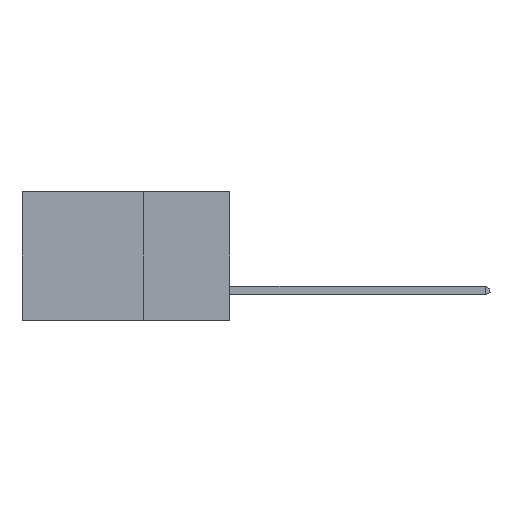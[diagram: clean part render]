
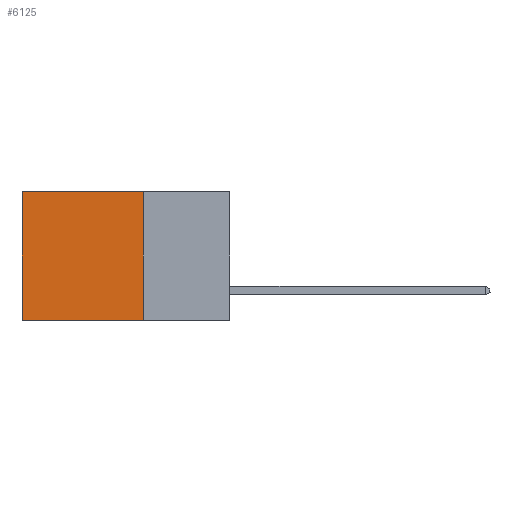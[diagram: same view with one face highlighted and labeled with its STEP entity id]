
A CAD part, left-side view. The second image highlights one B-rep face of the part: STEP entity #6125.
In plain terms, the highlighted planar face has unit normal (-1, 0, 0).
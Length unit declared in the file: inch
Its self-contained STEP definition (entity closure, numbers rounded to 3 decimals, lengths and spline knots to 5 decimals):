
#950 = CARTESIAN_POINT ( 'NONE',  ( 0.298, 0.6, 0. ) ) ;
#2033 = CARTESIAN_POINT ( 'NONE',  ( 0.298, 0.25, 0. ) ) ;
#2099 = DIRECTION ( 'NONE',  ( 0., 0., -1. ) ) ;
#2283 = LINE ( 'NONE', #5082, #8561 ) ;
#2630 = CARTESIAN_POINT ( 'NONE',  ( 0.298, 0.25, 0. ) ) ;
#2689 = DIRECTION ( 'NONE',  ( 0., 1., 0. ) ) ;
#2701 = VERTEX_POINT ( 'NONE', #8441 ) ;
#2992 = EDGE_CURVE ( 'NONE', #3090, #9941, #2283, .T. ) ;
#3090 = VERTEX_POINT ( 'NONE', #5691 ) ;
#3111 = VERTEX_POINT ( 'NONE', #10288 ) ;
#3938 = VECTOR ( 'NONE', #4282, 39.37008 ) ;
#4282 = DIRECTION ( 'NONE',  ( 0., 0., -1. ) ) ;
#4817 = EDGE_LOOP ( 'NONE', ( #6131, #19559, #10011, #19814 ) ) ;
#5082 = CARTESIAN_POINT ( 'NONE',  ( 0.298, 0.25, -0.37 ) ) ;
#5691 = CARTESIAN_POINT ( 'NONE',  ( 0.298, 0.25, -0.37 ) ) ;
#6125 = ADVANCED_FACE ( 'NONE', ( #16436 ), #11254, .F. ) ;
#6131 = ORIENTED_EDGE ( 'NONE', *, *, #15670, .T. ) ;
#6218 = EDGE_CURVE ( 'NONE', #2701, #3111, #8225, .T. ) ;
#7987 = VECTOR ( 'NONE', #2689, 39.37008 ) ;
#8225 = LINE ( 'NONE', #2630, #7987 ) ;
#8441 = CARTESIAN_POINT ( 'NONE',  ( 0.298, 0.25, 0. ) ) ;
#8561 = VECTOR ( 'NONE', #11490, 39.37008 ) ;
#9039 = AXIS2_PLACEMENT_3D ( 'NONE', #2033, #17479, #2099 ) ;
#9941 = VERTEX_POINT ( 'NONE', #12575 ) ;
#10011 = ORIENTED_EDGE ( 'NONE', *, *, #11499, .F. ) ;
#10288 = CARTESIAN_POINT ( 'NONE',  ( 0.298, 0.6, 0. ) ) ;
#11254 = PLANE ( 'NONE',  #9039 ) ;
#11490 = DIRECTION ( 'NONE',  ( 0., 1., 0. ) ) ;
#11499 = EDGE_CURVE ( 'NONE', #2701, #3090, #16681, .T. ) ;
#12081 = VECTOR ( 'NONE', #12682, 39.37008 ) ;
#12575 = CARTESIAN_POINT ( 'NONE',  ( 0.298, 0.6, -0.37 ) ) ;
#12682 = DIRECTION ( 'NONE',  ( 0., 0., -1. ) ) ;
#13126 = LINE ( 'NONE', #950, #3938 ) ;
#14192 = CARTESIAN_POINT ( 'NONE',  ( 0.298, 0.25, 0. ) ) ;
#15670 = EDGE_CURVE ( 'NONE', #3111, #9941, #13126, .T. ) ;
#16436 = FACE_OUTER_BOUND ( 'NONE', #4817, .T. ) ;
#16681 = LINE ( 'NONE', #14192, #12081 ) ;
#17479 = DIRECTION ( 'NONE',  ( 1., 0., 0. ) ) ;
#19559 = ORIENTED_EDGE ( 'NONE', *, *, #2992, .F. ) ;
#19814 = ORIENTED_EDGE ( 'NONE', *, *, #6218, .T. ) ;
